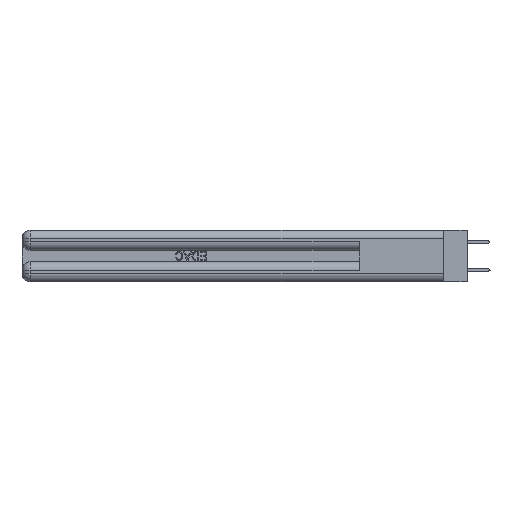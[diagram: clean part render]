
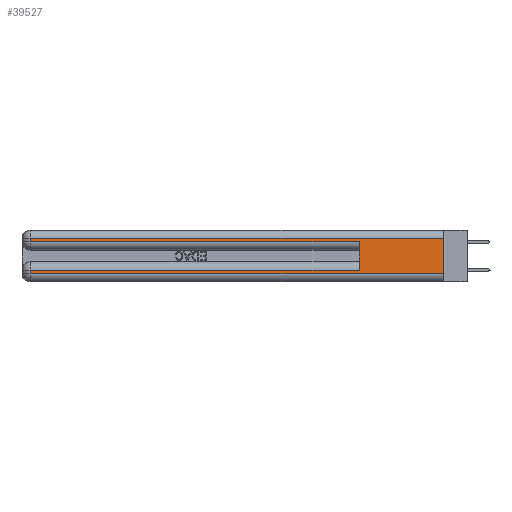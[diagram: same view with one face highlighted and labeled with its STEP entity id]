
A CAD part, left-side view. The second image highlights one B-rep face of the part: STEP entity #39527.
In plain terms, the highlighted planar face has unit normal (-1, 0, 0).
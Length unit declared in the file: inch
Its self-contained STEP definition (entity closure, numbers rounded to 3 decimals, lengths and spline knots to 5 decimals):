
#453 = VERTEX_POINT ( 'NONE', #43345 ) ;
#486 = VERTEX_POINT ( 'NONE', #13478 ) ;
#540 = VERTEX_POINT ( 'NONE', #36688 ) ;
#555 = DIRECTION ( 'NONE',  ( 0., 0., -1. ) ) ;
#868 = FACE_OUTER_BOUND ( 'NONE', #16903, .T. ) ;
#1011 = CARTESIAN_POINT ( 'NONE',  ( 0., 0.6, 0.085 ) ) ;
#2073 = VECTOR ( 'NONE', #4301, 39.37008 ) ;
#4088 = EDGE_CURVE ( 'NONE', #14401, #24139, #43029, .T. ) ;
#4301 = DIRECTION ( 'NONE',  ( 0., -1., 0. ) ) ;
#5022 = LINE ( 'NONE', #5946, #31919 ) ;
#5513 = CARTESIAN_POINT ( 'NONE',  ( 0., 0., 0.31 ) ) ;
#5946 = CARTESIAN_POINT ( 'NONE',  ( 0., 0., 0.085 ) ) ;
#7237 = VERTEX_POINT ( 'NONE', #11828 ) ;
#7626 = EDGE_CURVE ( 'NONE', #43215, #7237, #10984, .T. ) ;
#8046 = CARTESIAN_POINT ( 'NONE',  ( 0., 0., 0.37 ) ) ;
#8681 = VECTOR ( 'NONE', #33160, 39.37008 ) ;
#9382 = CARTESIAN_POINT ( 'NONE',  ( 0., 0.6, 0.145 ) ) ;
#10984 = LINE ( 'NONE', #20819, #2073 ) ;
#11604 = DIRECTION ( 'NONE',  ( 1., 0., 0. ) ) ;
#11828 = CARTESIAN_POINT ( 'NONE',  ( 0., 0., 0.06 ) ) ;
#12589 = CARTESIAN_POINT ( 'NONE',  ( 0., 2.94, 0.37 ) ) ;
#13314 = EDGE_CURVE ( 'NONE', #40396, #7237, #21607, .T. ) ;
#13478 = CARTESIAN_POINT ( 'NONE',  ( 0., 2.94, 0.31 ) ) ;
#13518 = ORIENTED_EDGE ( 'NONE', *, *, #13314, .F. ) ;
#14401 = VERTEX_POINT ( 'NONE', #1011 ) ;
#15018 = DIRECTION ( 'NONE',  ( 0., 0., -1. ) ) ;
#16903 = EDGE_LOOP ( 'NONE', ( #13518, #20202, #41171, #33396, #38255, #37819, #35140, #31659 ) ) ;
#18028 = LINE ( 'NONE', #27360, #34360 ) ;
#19090 = DIRECTION ( 'NONE',  ( 0., 1., 0. ) ) ;
#20202 = ORIENTED_EDGE ( 'NONE', *, *, #34516, .T. ) ;
#20291 = AXIS2_PLACEMENT_3D ( 'NONE', #8046, #11604, #15018 ) ;
#20462 = EDGE_CURVE ( 'NONE', #486, #453, #23229, .T. ) ;
#20819 = CARTESIAN_POINT ( 'NONE',  ( 0., 0., 0.06 ) ) ;
#21607 = LINE ( 'NONE', #38170, #25838 ) ;
#22454 = VECTOR ( 'NONE', #19090, 39.37008 ) ;
#23229 = LINE ( 'NONE', #12589, #32745 ) ;
#23828 = DIRECTION ( 'NONE',  ( 0., -1., 0. ) ) ;
#24053 = CARTESIAN_POINT ( 'NONE',  ( 0., 2.94, 0.06 ) ) ;
#24139 = VERTEX_POINT ( 'NONE', #39572 ) ;
#25116 = VECTOR ( 'NONE', #42337, 39.37008 ) ;
#25838 = VECTOR ( 'NONE', #31469, 39.37008 ) ;
#27360 = CARTESIAN_POINT ( 'NONE',  ( 0., 0., 0.285 ) ) ;
#28997 = CARTESIAN_POINT ( 'NONE',  ( 0., 0., 0.31 ) ) ;
#31469 = DIRECTION ( 'NONE',  ( 0., 0., -1. ) ) ;
#31659 = ORIENTED_EDGE ( 'NONE', *, *, #7626, .T. ) ;
#31919 = VECTOR ( 'NONE', #36133, 39.37008 ) ;
#32745 = VECTOR ( 'NONE', #555, 39.37008 ) ;
#32978 = LINE ( 'NONE', #28997, #22454 ) ;
#33160 = DIRECTION ( 'NONE',  ( 0., 0., -1. ) ) ;
#33396 = ORIENTED_EDGE ( 'NONE', *, *, #42440, .T. ) ;
#34360 = VECTOR ( 'NONE', #23828, 39.37008 ) ;
#34516 = EDGE_CURVE ( 'NONE', #40396, #486, #32978, .T. ) ;
#34581 = EDGE_CURVE ( 'NONE', #14401, #540, #5022, .T. ) ;
#35140 = ORIENTED_EDGE ( 'NONE', *, *, #36017, .T. ) ;
#36017 = EDGE_CURVE ( 'NONE', #540, #43215, #40771, .T. ) ;
#36133 = DIRECTION ( 'NONE',  ( 0., 1., 0. ) ) ;
#36688 = CARTESIAN_POINT ( 'NONE',  ( 0., 2.94, 0.085 ) ) ;
#37819 = ORIENTED_EDGE ( 'NONE', *, *, #34581, .T. ) ;
#37911 = PLANE ( 'NONE',  #20291 ) ;
#38170 = CARTESIAN_POINT ( 'NONE',  ( 0., 0., 0.37 ) ) ;
#38255 = ORIENTED_EDGE ( 'NONE', *, *, #4088, .F. ) ;
#39527 = ADVANCED_FACE ( 'NONE', ( #868 ), #37911, .F. ) ;
#39572 = CARTESIAN_POINT ( 'NONE',  ( 0., 0.6, 0.285 ) ) ;
#39889 = CARTESIAN_POINT ( 'NONE',  ( 0., 2.94, 0.37 ) ) ;
#40396 = VERTEX_POINT ( 'NONE', #5513 ) ;
#40771 = LINE ( 'NONE', #39889, #8681 ) ;
#41171 = ORIENTED_EDGE ( 'NONE', *, *, #20462, .T. ) ;
#42337 = DIRECTION ( 'NONE',  ( 0., 0., 1. ) ) ;
#42440 = EDGE_CURVE ( 'NONE', #453, #24139, #18028, .T. ) ;
#43029 = LINE ( 'NONE', #9382, #25116 ) ;
#43215 = VERTEX_POINT ( 'NONE', #24053 ) ;
#43345 = CARTESIAN_POINT ( 'NONE',  ( 0., 2.94, 0.285 ) ) ;
